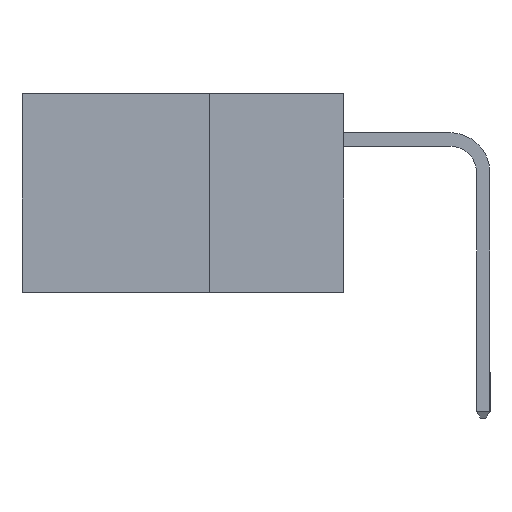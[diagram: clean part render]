
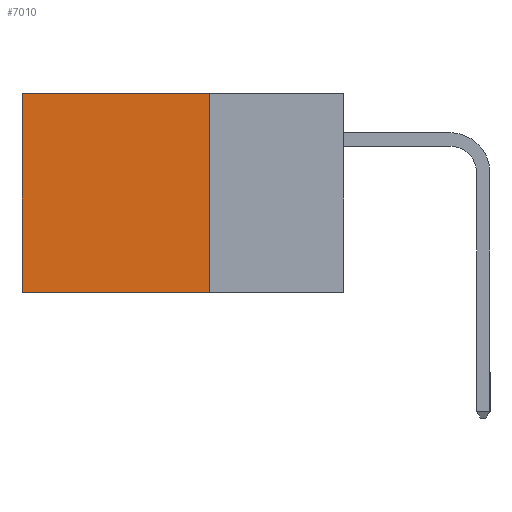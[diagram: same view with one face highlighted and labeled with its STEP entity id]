
A CAD part, left-side view. The second image highlights one B-rep face of the part: STEP entity #7010.
In plain terms, the highlighted planar face has unit normal (-1, 0, 0).
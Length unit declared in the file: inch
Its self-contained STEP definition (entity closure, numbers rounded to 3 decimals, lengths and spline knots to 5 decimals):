
#645 = DIRECTION ( 'NONE',  ( 0., 1., 0. ) ) ;
#734 = ORIENTED_EDGE ( 'NONE', *, *, #14309, .T. ) ;
#1423 = ORIENTED_EDGE ( 'NONE', *, *, #23392, .F. ) ;
#1725 = EDGE_CURVE ( 'NONE', #23123, #8454, #23248, .T. ) ;
#1936 = VECTOR ( 'NONE', #19964, 39.37008 ) ;
#2423 = FACE_OUTER_BOUND ( 'NONE', #11256, .T. ) ;
#2720 = VERTEX_POINT ( 'NONE', #23768 ) ;
#3330 = VERTEX_POINT ( 'NONE', #10937 ) ;
#5134 = CARTESIAN_POINT ( 'NONE',  ( 0.2615, 0.25, 0. ) ) ;
#5968 = CARTESIAN_POINT ( 'NONE',  ( 0.2615, 0.25, -0.37 ) ) ;
#6508 = VECTOR ( 'NONE', #9968, 39.37008 ) ;
#7010 = ADVANCED_FACE ( 'NONE', ( #2423 ), #13825, .F. ) ;
#7729 = LINE ( 'NONE', #5968, #6508 ) ;
#8454 = VERTEX_POINT ( 'NONE', #24760 ) ;
#9364 = ORIENTED_EDGE ( 'NONE', *, *, #22739, .F. ) ;
#9663 = CARTESIAN_POINT ( 'NONE',  ( 0.2615, 0.6, -0.37 ) ) ;
#9968 = DIRECTION ( 'NONE',  ( 0., 0., -1. ) ) ;
#10937 = CARTESIAN_POINT ( 'NONE',  ( 0.2615, 0.25, 0. ) ) ;
#11256 = EDGE_LOOP ( 'NONE', ( #14013, #9364, #1423, #734 ) ) ;
#12677 = LINE ( 'NONE', #20337, #17313 ) ;
#13825 = PLANE ( 'NONE',  #19802 ) ;
#14013 = ORIENTED_EDGE ( 'NONE', *, *, #1725, .T. ) ;
#14067 = DIRECTION ( 'NONE',  ( 1., 0., 0. ) ) ;
#14309 = EDGE_CURVE ( 'NONE', #3330, #23123, #18323, .T. ) ;
#17313 = VECTOR ( 'NONE', #645, 39.37008 ) ;
#18323 = LINE ( 'NONE', #5134, #1936 ) ;
#19146 = VECTOR ( 'NONE', #23611, 39.37008 ) ;
#19488 = CARTESIAN_POINT ( 'NONE',  ( 0.2615, 0.25, -0.37 ) ) ;
#19802 = AXIS2_PLACEMENT_3D ( 'NONE', #19488, #14067, #21740 ) ;
#19964 = DIRECTION ( 'NONE',  ( 0., 1., 0. ) ) ;
#20337 = CARTESIAN_POINT ( 'NONE',  ( 0.2615, 0.25, -0.37 ) ) ;
#21740 = DIRECTION ( 'NONE',  ( 0., 0., -1. ) ) ;
#22739 = EDGE_CURVE ( 'NONE', #2720, #8454, #12677, .T. ) ;
#23123 = VERTEX_POINT ( 'NONE', #23578 ) ;
#23248 = LINE ( 'NONE', #9663, #19146 ) ;
#23392 = EDGE_CURVE ( 'NONE', #3330, #2720, #7729, .T. ) ;
#23578 = CARTESIAN_POINT ( 'NONE',  ( 0.2615, 0.6, 0. ) ) ;
#23611 = DIRECTION ( 'NONE',  ( 0., 0., -1. ) ) ;
#23768 = CARTESIAN_POINT ( 'NONE',  ( 0.2615, 0.25, -0.37 ) ) ;
#24760 = CARTESIAN_POINT ( 'NONE',  ( 0.2615, 0.6, -0.37 ) ) ;
